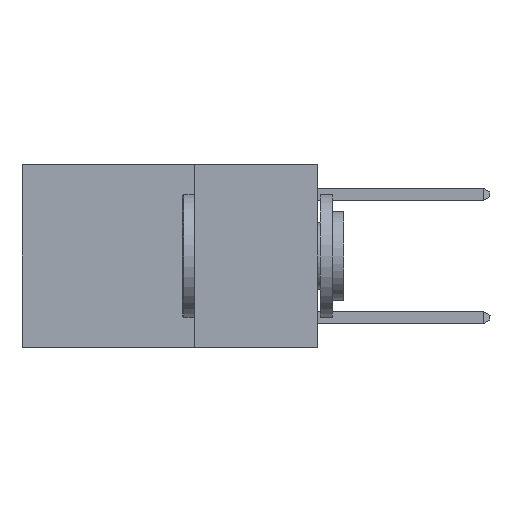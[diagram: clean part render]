
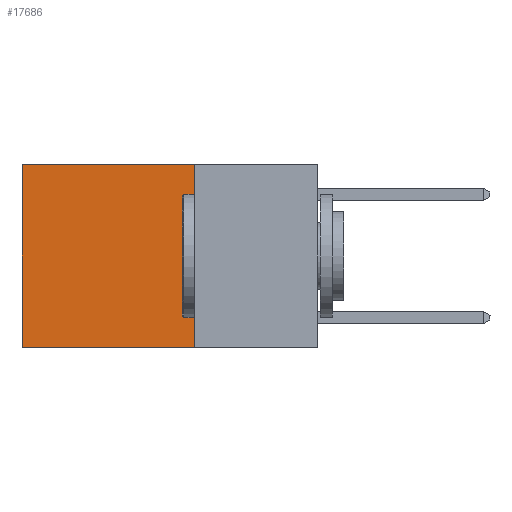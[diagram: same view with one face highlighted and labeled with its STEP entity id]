
A CAD part, left-side view. The second image highlights one B-rep face of the part: STEP entity #17686.
In plain terms, the highlighted planar face has unit normal (-1, 0, 0).
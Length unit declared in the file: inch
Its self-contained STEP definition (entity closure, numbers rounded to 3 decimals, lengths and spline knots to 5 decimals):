
#1366 = EDGE_CURVE ( 'NONE', #12115, #5557, #4577, .T. ) ;
#2152 = VECTOR ( 'NONE', #19119, 39.37008 ) ;
#2541 = CARTESIAN_POINT ( 'NONE',  ( 0.2625, 0.25, -0.37 ) ) ;
#2602 = VECTOR ( 'NONE', #7513, 39.37008 ) ;
#2894 = FACE_OUTER_BOUND ( 'NONE', #12619, .T. ) ;
#3711 = EDGE_CURVE ( 'NONE', #26113, #12865, #3932, .T. ) ;
#3866 = ORIENTED_EDGE ( 'NONE', *, *, #3711, .T. ) ;
#3932 = LINE ( 'NONE', #12071, #2602 ) ;
#4577 = LINE ( 'NONE', #25489, #13772 ) ;
#5557 = VERTEX_POINT ( 'NONE', #2541 ) ;
#6716 = EDGE_CURVE ( 'NONE', #12115, #26113, #15344, .T. ) ;
#7099 = CARTESIAN_POINT ( 'NONE',  ( 0.2625, 0.25, 0. ) ) ;
#7513 = DIRECTION ( 'NONE',  ( 0., 0., -1. ) ) ;
#10566 = ORIENTED_EDGE ( 'NONE', *, *, #20987, .F. ) ;
#12071 = CARTESIAN_POINT ( 'NONE',  ( 0.2625, 0.6, 0. ) ) ;
#12115 = VERTEX_POINT ( 'NONE', #24270 ) ;
#12619 = EDGE_LOOP ( 'NONE', ( #3866, #10566, #27783, #22533 ) ) ;
#12840 = LINE ( 'NONE', #19562, #27804 ) ;
#12865 = VERTEX_POINT ( 'NONE', #16596 ) ;
#13772 = VECTOR ( 'NONE', #16877, 39.37008 ) ;
#15344 = LINE ( 'NONE', #21014, #2152 ) ;
#16596 = CARTESIAN_POINT ( 'NONE',  ( 0.2625, 0.6, -0.37 ) ) ;
#16877 = DIRECTION ( 'NONE',  ( 0., 0., -1. ) ) ;
#17686 = ADVANCED_FACE ( 'NONE', ( #2894 ), #17907, .F. ) ;
#17907 = PLANE ( 'NONE',  #23319 ) ;
#19119 = DIRECTION ( 'NONE',  ( 0., 1., 0. ) ) ;
#19562 = CARTESIAN_POINT ( 'NONE',  ( 0.2625, 0.25, -0.37 ) ) ;
#20987 = EDGE_CURVE ( 'NONE', #5557, #12865, #12840, .T. ) ;
#21014 = CARTESIAN_POINT ( 'NONE',  ( 0.2625, 0.25, 0. ) ) ;
#21050 = DIRECTION ( 'NONE',  ( 0., 0., -1. ) ) ;
#22533 = ORIENTED_EDGE ( 'NONE', *, *, #6716, .T. ) ;
#22919 = CARTESIAN_POINT ( 'NONE',  ( 0.2625, 0.6, 0. ) ) ;
#23319 = AXIS2_PLACEMENT_3D ( 'NONE', #7099, #26658, #21050 ) ;
#24270 = CARTESIAN_POINT ( 'NONE',  ( 0.2625, 0.25, 0. ) ) ;
#25489 = CARTESIAN_POINT ( 'NONE',  ( 0.2625, 0.25, 0. ) ) ;
#26113 = VERTEX_POINT ( 'NONE', #22919 ) ;
#26658 = DIRECTION ( 'NONE',  ( 1., 0., 0. ) ) ;
#27783 = ORIENTED_EDGE ( 'NONE', *, *, #1366, .F. ) ;
#27804 = VECTOR ( 'NONE', #28002, 39.37008 ) ;
#28002 = DIRECTION ( 'NONE',  ( 0., 1., 0. ) ) ;
